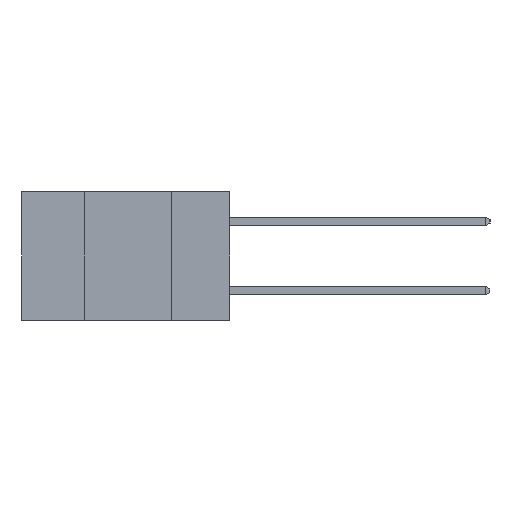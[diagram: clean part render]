
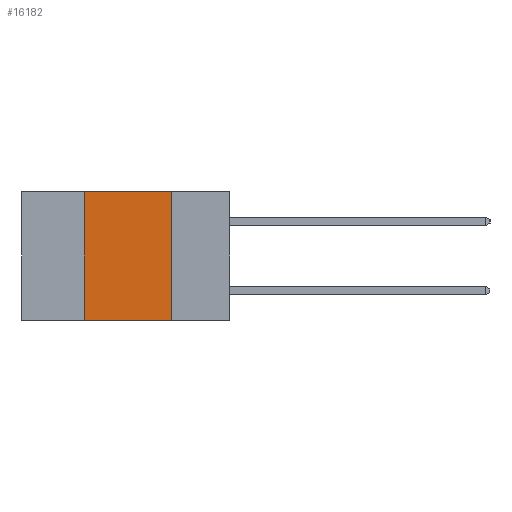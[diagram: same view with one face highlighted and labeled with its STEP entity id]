
A CAD part, left-side view. The second image highlights one B-rep face of the part: STEP entity #16182.
In plain terms, the highlighted planar face has unit normal (-1, 0, 0).
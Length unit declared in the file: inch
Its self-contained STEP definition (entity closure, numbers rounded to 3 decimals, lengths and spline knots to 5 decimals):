
#843 = CARTESIAN_POINT ( 'NONE',  ( 0., 0.42, -0.37 ) ) ;
#1191 = DIRECTION ( 'NONE',  ( 0., 0., -1. ) ) ;
#1676 = EDGE_LOOP ( 'NONE', ( #22551, #8559, #18868, #4761 ) ) ;
#1876 = CARTESIAN_POINT ( 'NONE',  ( 0., 0.17, 0. ) ) ;
#2706 = DIRECTION ( 'NONE',  ( 0., 0., 1. ) ) ;
#3661 = VECTOR ( 'NONE', #1191, 39.37008 ) ;
#3851 = FACE_OUTER_BOUND ( 'NONE', #1676, .T. ) ;
#4761 = ORIENTED_EDGE ( 'NONE', *, *, #19757, .T. ) ;
#4948 = CARTESIAN_POINT ( 'NONE',  ( 0., 0.6, 0. ) ) ;
#6650 = CARTESIAN_POINT ( 'NONE',  ( 0., 0.6, -0.37 ) ) ;
#8025 = VECTOR ( 'NONE', #8523, 39.37008 ) ;
#8523 = DIRECTION ( 'NONE',  ( 0., -1., 0. ) ) ;
#8559 = ORIENTED_EDGE ( 'NONE', *, *, #10742, .F. ) ;
#8629 = LINE ( 'NONE', #6650, #8025 ) ;
#9259 = VECTOR ( 'NONE', #17839, 39.37008 ) ;
#9838 = LINE ( 'NONE', #4948, #9259 ) ;
#10436 = DIRECTION ( 'NONE',  ( 1., 0., 0. ) ) ;
#10742 = EDGE_CURVE ( 'NONE', #12770, #16917, #9838, .T. ) ;
#11946 = EDGE_CURVE ( 'NONE', #16917, #17908, #23714, .T. ) ;
#12111 = LINE ( 'NONE', #843, #21236 ) ;
#12770 = VERTEX_POINT ( 'NONE', #18075 ) ;
#15111 = AXIS2_PLACEMENT_3D ( 'NONE', #21345, #10436, #23150 ) ;
#15258 = CARTESIAN_POINT ( 'NONE',  ( 0., 0.42, -0.37 ) ) ;
#15942 = VERTEX_POINT ( 'NONE', #15258 ) ;
#16182 = ADVANCED_FACE ( 'NONE', ( #3851 ), #23072, .F. ) ;
#16917 = VERTEX_POINT ( 'NONE', #1876 ) ;
#17839 = DIRECTION ( 'NONE',  ( 0., -1., 0. ) ) ;
#17908 = VERTEX_POINT ( 'NONE', #21434 ) ;
#18075 = CARTESIAN_POINT ( 'NONE',  ( 0., 0.42, 0. ) ) ;
#18868 = ORIENTED_EDGE ( 'NONE', *, *, #20953, .F. ) ;
#19757 = EDGE_CURVE ( 'NONE', #15942, #17908, #8629, .T. ) ;
#20953 = EDGE_CURVE ( 'NONE', #15942, #12770, #12111, .T. ) ;
#21236 = VECTOR ( 'NONE', #2706, 39.37008 ) ;
#21345 = CARTESIAN_POINT ( 'NONE',  ( 0., 0.6, 0. ) ) ;
#21434 = CARTESIAN_POINT ( 'NONE',  ( 0., 0.17, -0.37 ) ) ;
#22551 = ORIENTED_EDGE ( 'NONE', *, *, #11946, .F. ) ;
#23072 = PLANE ( 'NONE',  #15111 ) ;
#23150 = DIRECTION ( 'NONE',  ( 0., 0., -1. ) ) ;
#23161 = CARTESIAN_POINT ( 'NONE',  ( 0., 0.17, -0.37 ) ) ;
#23714 = LINE ( 'NONE', #23161, #3661 ) ;
